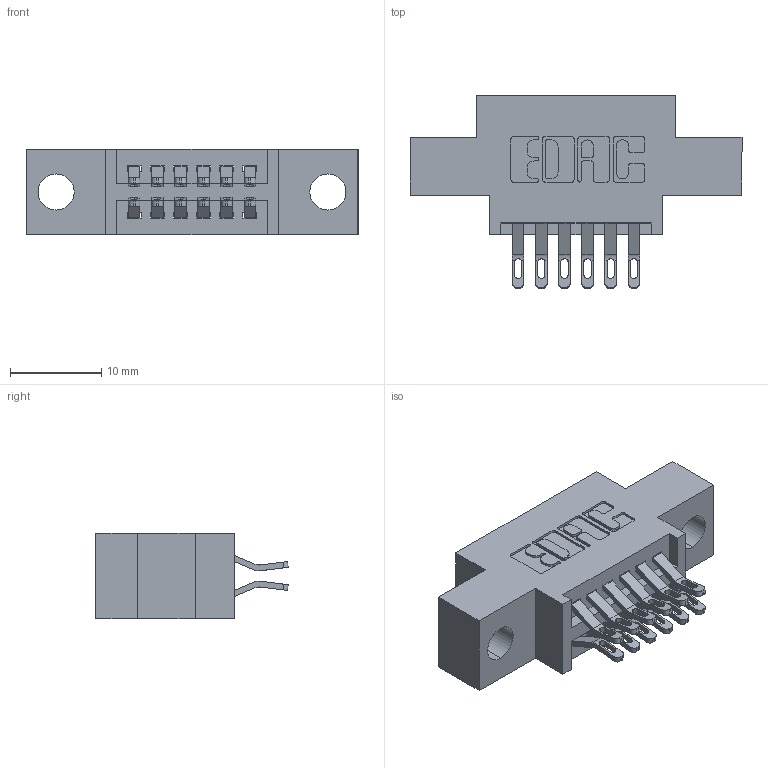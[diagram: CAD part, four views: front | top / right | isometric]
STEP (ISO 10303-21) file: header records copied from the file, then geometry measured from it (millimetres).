
FILE_DESCRIPTION (( 'STEP AP203' ), '1' );
FILE_NAME ('395-012-555-804.STEP', '2018-11-05T18:59:22', ( '' ), ( '' ), 'SwSTEP 2.0', 'SolidWorks 2016', '' );
FILE_SCHEMA (( 'CONFIG_CONTROL_DESIGN' ));
Length unit declared in the file: inch
Products named in the file (3): 395-012-555-804; 345 Part_0.170 Offset - 0.156 Dia-TH; 345-292-001_555 Tail
Assembly tree (13 placements, depth 2):
  395-012-555-804
    345 Part_0.170 Offset - 0.156 Dia-TH
    345-292-001_555 Tail  x12
Bounding box: 36.45 x 21.13 x 9.4 mm (x, y, z)
Volume: 3040.1 mm3; surface area: 3876.2 mm2
Topology: 13 solids, 13 shells, 802 faces, 2477 edges, 1650 vertices
Faces by surface type: plane 456, cylinder 346
Entity records: 10015 total; most frequent: CARTESIAN_POINT 1750, ORIENTED_EDGE 1654, DIRECTION 1555, EDGE_CURVE 827, VECTOR 651, LINE 651, VERTEX_POINT 550, AXIS2_PLACEMENT_3D 452
